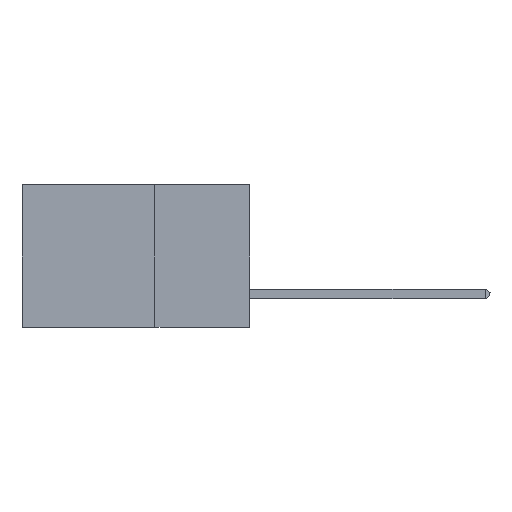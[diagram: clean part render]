
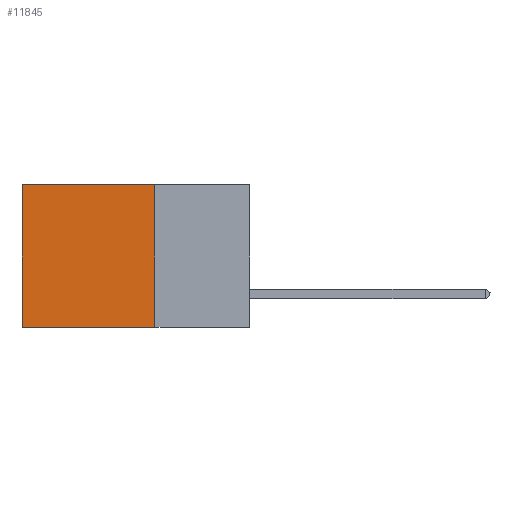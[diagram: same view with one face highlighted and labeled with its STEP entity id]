
A CAD part, left-side view. The second image highlights one B-rep face of the part: STEP entity #11845.
In plain terms, the highlighted planar face has unit normal (-1, 0, 0).
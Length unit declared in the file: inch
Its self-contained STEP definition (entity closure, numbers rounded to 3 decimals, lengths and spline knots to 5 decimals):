
#255 = CARTESIAN_POINT ( 'NONE',  ( 0.2875, 0.6, -0.375 ) ) ;
#603 = DIRECTION ( 'NONE',  ( 0., 0., -1. ) ) ;
#1371 = VECTOR ( 'NONE', #14894, 39.37008 ) ;
#1399 = ORIENTED_EDGE ( 'NONE', *, *, #8357, .T. ) ;
#2722 = VECTOR ( 'NONE', #14301, 39.37008 ) ;
#2828 = CARTESIAN_POINT ( 'NONE',  ( 0.2875, 0.25, -0.375 ) ) ;
#4078 = CARTESIAN_POINT ( 'NONE',  ( 0.2875, 0.25, -0.375 ) ) ;
#5118 = EDGE_LOOP ( 'NONE', ( #1399, #5318, #10246, #20123 ) ) ;
#5318 = ORIENTED_EDGE ( 'NONE', *, *, #7865, .F. ) ;
#5419 = EDGE_CURVE ( 'NONE', #12813, #7568, #5521, .T. ) ;
#5521 = LINE ( 'NONE', #10805, #21773 ) ;
#6946 = LINE ( 'NONE', #12119, #12267 ) ;
#7490 = CARTESIAN_POINT ( 'NONE',  ( 0.2875, 0.25, 0. ) ) ;
#7568 = VERTEX_POINT ( 'NONE', #14986 ) ;
#7865 = EDGE_CURVE ( 'NONE', #7568, #9771, #16588, .T. ) ;
#8357 = EDGE_CURVE ( 'NONE', #19362, #9771, #10440, .T. ) ;
#9771 = VERTEX_POINT ( 'NONE', #255 ) ;
#10246 = ORIENTED_EDGE ( 'NONE', *, *, #5419, .F. ) ;
#10440 = LINE ( 'NONE', #14964, #1371 ) ;
#10805 = CARTESIAN_POINT ( 'NONE',  ( 0.2875, 0.25, -0.375 ) ) ;
#11084 = FACE_OUTER_BOUND ( 'NONE', #5118, .T. ) ;
#11845 = ADVANCED_FACE ( 'NONE', ( #11084 ), #16626, .F. ) ;
#12119 = CARTESIAN_POINT ( 'NONE',  ( 0.2875, 0.25, 0. ) ) ;
#12267 = VECTOR ( 'NONE', #16511, 39.37008 ) ;
#12813 = VERTEX_POINT ( 'NONE', #7490 ) ;
#14301 = DIRECTION ( 'NONE',  ( 0., 1., 0. ) ) ;
#14894 = DIRECTION ( 'NONE',  ( 0., 0., -1. ) ) ;
#14964 = CARTESIAN_POINT ( 'NONE',  ( 0.2875, 0.6, -0.375 ) ) ;
#14986 = CARTESIAN_POINT ( 'NONE',  ( 0.2875, 0.25, -0.375 ) ) ;
#15062 = DIRECTION ( 'NONE',  ( 0., 0., -1. ) ) ;
#16511 = DIRECTION ( 'NONE',  ( 0., 1., 0. ) ) ;
#16546 = DIRECTION ( 'NONE',  ( 1., 0., 0. ) ) ;
#16588 = LINE ( 'NONE', #4078, #2722 ) ;
#16626 = PLANE ( 'NONE',  #20501 ) ;
#17166 = CARTESIAN_POINT ( 'NONE',  ( 0.2875, 0.6, 0. ) ) ;
#17466 = EDGE_CURVE ( 'NONE', #12813, #19362, #6946, .T. ) ;
#19362 = VERTEX_POINT ( 'NONE', #17166 ) ;
#20123 = ORIENTED_EDGE ( 'NONE', *, *, #17466, .T. ) ;
#20501 = AXIS2_PLACEMENT_3D ( 'NONE', #2828, #16546, #15062 ) ;
#21773 = VECTOR ( 'NONE', #603, 39.37008 ) ;
